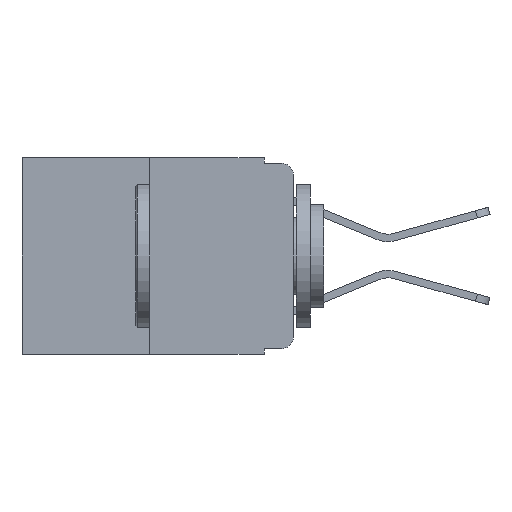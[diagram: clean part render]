
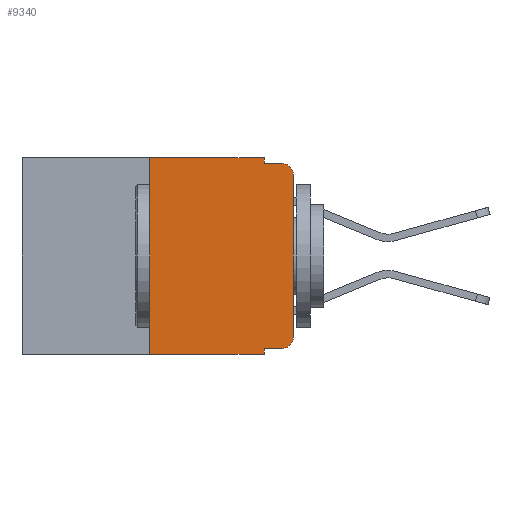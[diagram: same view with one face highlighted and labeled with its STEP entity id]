
A CAD part, left-side view. The second image highlights one B-rep face of the part: STEP entity #9340.
In plain terms, the highlighted planar face has unit normal (-1, 0, 0).
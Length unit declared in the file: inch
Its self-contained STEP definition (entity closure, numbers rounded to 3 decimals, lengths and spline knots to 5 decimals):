
#84 = DIRECTION ( 'NONE',  ( 0., 0., -1. ) ) ;
#484 = LINE ( 'NONE', #21589, #11057 ) ;
#688 = DIRECTION ( 'NONE',  ( 0., -1., 0. ) ) ;
#974 = VERTEX_POINT ( 'NONE', #9717 ) ;
#1320 = VECTOR ( 'NONE', #22084, 39.37008 ) ;
#1969 = VECTOR ( 'NONE', #4387, 39.37008 ) ;
#2182 = AXIS2_PLACEMENT_3D ( 'NONE', #3936, #16748, #5841 ) ;
#2511 = CARTESIAN_POINT ( 'NONE',  ( 0., 0.051, -0.343 ) ) ;
#2729 = VECTOR ( 'NONE', #21842, 39.37008 ) ;
#2871 = CARTESIAN_POINT ( 'NONE',  ( 0., 0., 0. ) ) ;
#3574 = CARTESIAN_POINT ( 'NONE',  ( 0., 0.051, -0.333 ) ) ;
#3810 = EDGE_CURVE ( 'NONE', #4073, #19068, #8821, .T. ) ;
#3936 = CARTESIAN_POINT ( 'NONE',  ( 0., 0.02, -0.03 ) ) ;
#3959 = ORIENTED_EDGE ( 'NONE', *, *, #5764, .F. ) ;
#4073 = VERTEX_POINT ( 'NONE', #4670 ) ;
#4245 = ORIENTED_EDGE ( 'NONE', *, *, #14612, .F. ) ;
#4312 = CARTESIAN_POINT ( 'NONE',  ( 0., 0., -0.313 ) ) ;
#4387 = DIRECTION ( 'NONE',  ( 0., -1., 0. ) ) ;
#4670 = CARTESIAN_POINT ( 'NONE',  ( 0., 0., -0.03 ) ) ;
#4888 = VERTEX_POINT ( 'NONE', #3574 ) ;
#5230 = EDGE_CURVE ( 'NONE', #13979, #10489, #12228, .T. ) ;
#5764 = EDGE_CURVE ( 'NONE', #4888, #10489, #484, .T. ) ;
#5841 = DIRECTION ( 'NONE',  ( 0., 0., -1. ) ) ;
#6091 = CARTESIAN_POINT ( 'NONE',  ( 0., 0.02, -0.01 ) ) ;
#6577 = ORIENTED_EDGE ( 'NONE', *, *, #19866, .F. ) ;
#7333 = LINE ( 'NONE', #2871, #21614 ) ;
#7564 = LINE ( 'NONE', #11764, #1969 ) ;
#7696 = CARTESIAN_POINT ( 'NONE',  ( 0., 0.02, -0.313 ) ) ;
#7710 = LINE ( 'NONE', #9381, #2729 ) ;
#8213 = CARTESIAN_POINT ( 'NONE',  ( 0., 0.473, 0. ) ) ;
#8413 = CARTESIAN_POINT ( 'NONE',  ( 0., 0.051, 0. ) ) ;
#8821 = CIRCLE ( 'NONE', #2182, 0.02 ) ;
#8923 = ORIENTED_EDGE ( 'NONE', *, *, #17290, .T. ) ;
#9340 = ADVANCED_FACE ( 'NONE', ( #11400 ), #18977, .F. ) ;
#9381 = CARTESIAN_POINT ( 'NONE',  ( 0., 0.25, 0. ) ) ;
#9557 = DIRECTION ( 'NONE',  ( 0., 0., -1. ) ) ;
#9717 = CARTESIAN_POINT ( 'NONE',  ( 0., 0.051, -0.01 ) ) ;
#9736 = ORIENTED_EDGE ( 'NONE', *, *, #17723, .T. ) ;
#10013 = EDGE_CURVE ( 'NONE', #17294, #4073, #7333, .T. ) ;
#10036 = ORIENTED_EDGE ( 'NONE', *, *, #22403, .F. ) ;
#10054 = DIRECTION ( 'NONE',  ( 0., 0., -1. ) ) ;
#10489 = VERTEX_POINT ( 'NONE', #2511 ) ;
#10808 = CARTESIAN_POINT ( 'NONE',  ( 0., 0.473, 0. ) ) ;
#11057 = VECTOR ( 'NONE', #19843, 39.37008 ) ;
#11274 = LINE ( 'NONE', #16815, #1320 ) ;
#11400 = FACE_OUTER_BOUND ( 'NONE', #17043, .T. ) ;
#11669 = VECTOR ( 'NONE', #688, 39.37008 ) ;
#11764 = CARTESIAN_POINT ( 'NONE',  ( 0., 0.051, -0.333 ) ) ;
#12228 = LINE ( 'NONE', #13731, #11669 ) ;
#13166 = CARTESIAN_POINT ( 'NONE',  ( 0., 0.051, 0. ) ) ;
#13640 = EDGE_CURVE ( 'NONE', #23036, #974, #14896, .T. ) ;
#13649 = VECTOR ( 'NONE', #23177, 39.37008 ) ;
#13731 = CARTESIAN_POINT ( 'NONE',  ( 0., 0.473, -0.343 ) ) ;
#13868 = AXIS2_PLACEMENT_3D ( 'NONE', #7696, #20246, #9557 ) ;
#13979 = VERTEX_POINT ( 'NONE', #21164 ) ;
#14612 = EDGE_CURVE ( 'NONE', #13979, #18864, #7710, .T. ) ;
#14672 = CARTESIAN_POINT ( 'NONE',  ( 0., 0.25, 0. ) ) ;
#14896 = LINE ( 'NONE', #13166, #19561 ) ;
#14962 = AXIS2_PLACEMENT_3D ( 'NONE', #8213, #20719, #10054 ) ;
#15187 = ORIENTED_EDGE ( 'NONE', *, *, #5230, .T. ) ;
#16748 = DIRECTION ( 'NONE',  ( -1., 0., 0. ) ) ;
#16815 = CARTESIAN_POINT ( 'NONE',  ( 0., 0.051, -0.01 ) ) ;
#17043 = EDGE_LOOP ( 'NONE', ( #17355, #21995, #10036, #20084, #6577, #4245, #15187, #3959, #8923, #9736 ) ) ;
#17290 = EDGE_CURVE ( 'NONE', #4888, #18680, #7564, .T. ) ;
#17294 = VERTEX_POINT ( 'NONE', #4312 ) ;
#17355 = ORIENTED_EDGE ( 'NONE', *, *, #10013, .T. ) ;
#17504 = DIRECTION ( 'NONE',  ( 0., 0., 1. ) ) ;
#17685 = CARTESIAN_POINT ( 'NONE',  ( 0., 0.02, -0.333 ) ) ;
#17723 = EDGE_CURVE ( 'NONE', #18680, #17294, #20720, .T. ) ;
#18680 = VERTEX_POINT ( 'NONE', #17685 ) ;
#18864 = VERTEX_POINT ( 'NONE', #14672 ) ;
#18977 = PLANE ( 'NONE',  #14962 ) ;
#19068 = VERTEX_POINT ( 'NONE', #6091 ) ;
#19561 = VECTOR ( 'NONE', #84, 39.37008 ) ;
#19843 = DIRECTION ( 'NONE',  ( 0., 0., -1. ) ) ;
#19866 = EDGE_CURVE ( 'NONE', #18864, #23036, #22455, .T. ) ;
#20084 = ORIENTED_EDGE ( 'NONE', *, *, #13640, .F. ) ;
#20246 = DIRECTION ( 'NONE',  ( -1., 0., 0. ) ) ;
#20719 = DIRECTION ( 'NONE',  ( 1., 0., 0. ) ) ;
#20720 = CIRCLE ( 'NONE', #13868, 0.02 ) ;
#21164 = CARTESIAN_POINT ( 'NONE',  ( 0., 0.25, -0.343 ) ) ;
#21589 = CARTESIAN_POINT ( 'NONE',  ( 0., 0.051, 0. ) ) ;
#21614 = VECTOR ( 'NONE', #17504, 39.37008 ) ;
#21842 = DIRECTION ( 'NONE',  ( 0., 0., 1. ) ) ;
#21995 = ORIENTED_EDGE ( 'NONE', *, *, #3810, .T. ) ;
#22084 = DIRECTION ( 'NONE',  ( 0., -1., 0. ) ) ;
#22403 = EDGE_CURVE ( 'NONE', #974, #19068, #11274, .T. ) ;
#22455 = LINE ( 'NONE', #10808, #13649 ) ;
#23036 = VERTEX_POINT ( 'NONE', #8413 ) ;
#23177 = DIRECTION ( 'NONE',  ( 0., -1., 0. ) ) ;
